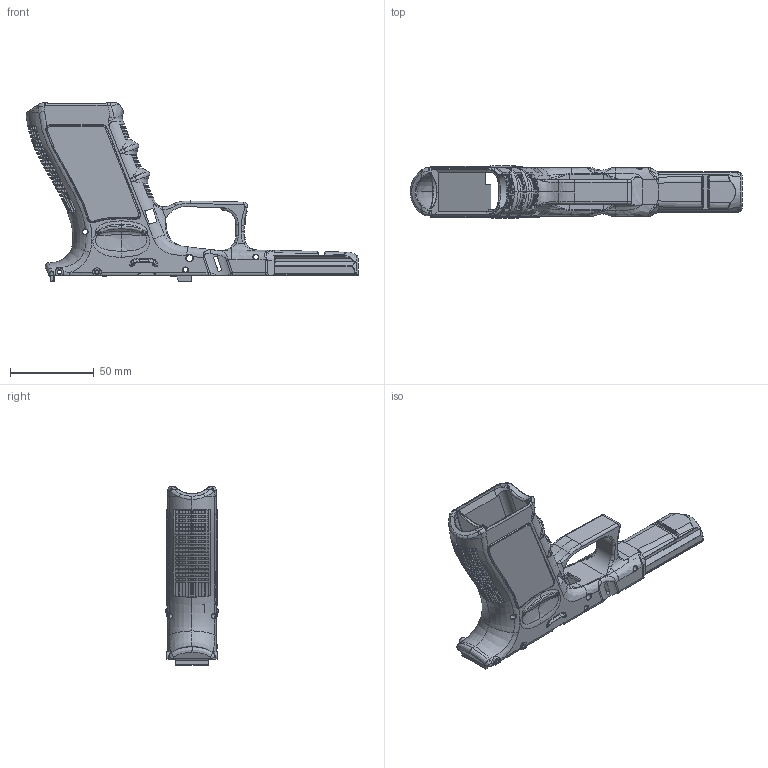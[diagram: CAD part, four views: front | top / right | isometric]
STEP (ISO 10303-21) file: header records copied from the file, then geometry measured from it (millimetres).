
FILE_DESCRIPTION(/* description */ (''),/* implementation_level */ '2;1');
FILE_NAME(/* name */ 'full_mod10_kill_embellish3_reset_hx v1.step',/* time_stamp */ '2020-01-08T14:39:54-08:00',/* author */ (''),/* organization */ (''),/* preprocessor_version */ 'ST-DEVELOPER v18',/* originating_system */ 'Autodesk Translation Framework v8.12.0.6',/* authorisation */ '');
FILE_SCHEMA (('AUTOMOTIVE_DESIGN { 1 0 10303 214 3 1 1 }'));
Products named in the file (2): full_mod10_kill_embellish3_reset_hx; mod10
Assembly tree (1 placements, depth 2):
  full_mod10_kill_embellish3_reset_hx
    mod10
Bounding box: 197.79 x 31.4 x 106.5 mm (x, y, z)
Volume: 80453.3 mm3; surface area: 51556.5 mm2
Topology: 1 solids, 1 shells, 2421 faces, 7017 edges, 4575 vertices
Faces by surface type: bspline 1063, plane 863, cylinder 419, cone 35, torus 27, sphere 14
Full cylindrical faces by diameter (mm): 2.25 x4, 2.3 x4, 3 x6, 4 x2
Entity records: 185921 total; most frequent: CARTESIAN_POINT 128411, ORIENTED_EDGE 13998, DIRECTION 9786, EDGE_CURVE 6999, VERTEX_POINT 4575, AXIS2_PLACEMENT_3D 3549, LINE 2688, VECTOR 2688
